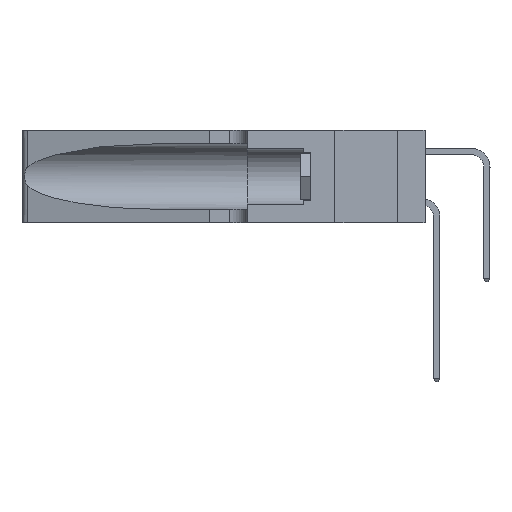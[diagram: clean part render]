
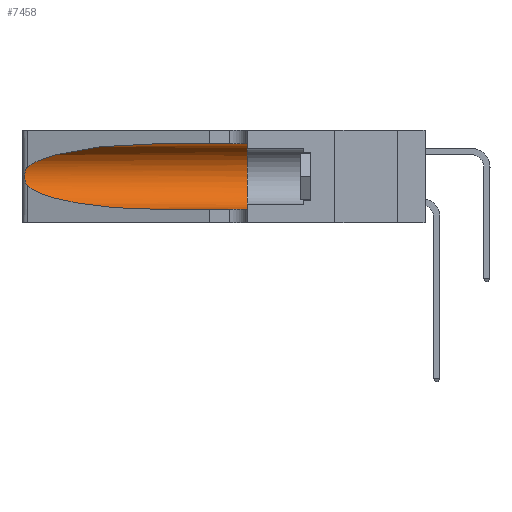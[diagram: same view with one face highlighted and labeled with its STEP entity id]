
A CAD part, left-side view. The second image highlights one B-rep face of the part: STEP entity #7458.
In plain terms, the highlighted cylindrical face has radius 3.308 mm (diameter 6.617 mm), a partial arc.
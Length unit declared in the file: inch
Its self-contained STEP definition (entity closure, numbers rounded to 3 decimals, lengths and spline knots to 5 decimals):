
#103 = CARTESIAN_POINT ( 'NONE',  ( 0.1305, 1.61858, 0.05475 ) ) ;
#185 = DIRECTION ( 'NONE',  ( 0., -1., 0. ) ) ;
#782 = B_SPLINE_CURVE_WITH_KNOTS ( 'NONE', 3,
 ( #19100, #15701, #3458, #15785, #5292, #17506, #7120, #19171, #8895, #20859, #10693, #22565, #12404, #1718 ),
 .UNSPECIFIED., .F., .F.,
 ( 4, 2, 2, 2, 2, 2, 4 ),
 ( 0., 0.00027, 0.00053, 0.00107, 0.0016, 0.00187, 0.00214 ),
 .UNSPECIFIED. ) ;
#835 = DIRECTION ( 'NONE',  ( 0., 0., -1. ) ) ;
#1412 = VERTEX_POINT ( 'NONE', #7590 ) ;
#1500 = CARTESIAN_POINT ( 'NONE',  ( 0.1305, 0.35, 0.31525 ) ) ;
#1718 = CARTESIAN_POINT ( 'NONE',  ( 0.25487, 1.22718, 0.14631 ) ) ;
#2585 = DIRECTION ( 'NONE',  ( 0., 1., 0. ) ) ;
#3244 =( BOUNDED_CURVE ( )  B_SPLINE_CURVE ( 3, ( #16791, #18538, #8221, #20223 ),
 .UNSPECIFIED., .F., .F. ) 
 B_SPLINE_CURVE_WITH_KNOTS ( ( 4, 4 ),
 ( 3.44316, 4.71239 ),
 .UNSPECIFIED. ) 
 CURVE ( )  GEOMETRIC_REPRESENTATION_ITEM ( )  RATIONAL_B_SPLINE_CURVE ( ( 1., 0.87, 0.87, 1. ) ) 
 REPRESENTATION_ITEM ( '' )  );
#3458 = CARTESIAN_POINT ( 'NONE',  ( 0.25639, 1.23184, 0.21858 ) ) ;
#3823 = EDGE_CURVE ( 'NONE', #5404, #13531, #11294, .T. ) ;
#4057 = EDGE_CURVE ( 'NONE', #19963, #5404, #20044, .T. ) ;
#4333 = EDGE_CURVE ( 'NONE', #20969, #13531, #15296, .T. ) ;
#4766 = CARTESIAN_POINT ( 'NONE',  ( 0.25487, 1.22718, 0.14631 ) ) ;
#4829 = CARTESIAN_POINT ( 'NONE',  ( 0.1305, 0.72297, 0.05475 ) ) ;
#4908 = ORIENTED_EDGE ( 'NONE', *, *, #4333, .T. ) ;
#4962 = DIRECTION ( 'NONE',  ( 0., -1., 0. ) ) ;
#5292 = CARTESIAN_POINT ( 'NONE',  ( 0.25854, 1.2359, 0.20912 ) ) ;
#5404 = VERTEX_POINT ( 'NONE', #1500 ) ;
#5486 = EDGE_CURVE ( 'NONE', #19963, #1412, #5718, .T. ) ;
#5718 =( BOUNDED_CURVE ( )  B_SPLINE_CURVE ( 3, ( #18509, #8193, #20181, #9987 ),
 .UNSPECIFIED., .F., .T. ) 
 B_SPLINE_CURVE_WITH_KNOTS ( ( 4, 4 ),
 ( 1.5708, 2.84003 ),
 .UNSPECIFIED. ) 
 CURVE ( )  GEOMETRIC_REPRESENTATION_ITEM ( )  RATIONAL_B_SPLINE_CURVE ( ( 1., 0.87, 0.87, 1. ) ) 
 REPRESENTATION_ITEM ( '' )  );
#6561 = VECTOR ( 'NONE', #185, 39.37008 ) ;
#6978 = ORIENTED_EDGE ( 'NONE', *, *, #3823, .F. ) ;
#7120 = CARTESIAN_POINT ( 'NONE',  ( 0.26075, 1.23896, 0.19203 ) ) ;
#7458 = ADVANCED_FACE ( 'NONE', ( #16131 ), #15579, .F. ) ;
#7590 = CARTESIAN_POINT ( 'NONE',  ( 0.25487, 1.22718, 0.22369 ) ) ;
#8193 = CARTESIAN_POINT ( 'NONE',  ( 0.18966, 0.96281, 0.31525 ) ) ;
#8221 = CARTESIAN_POINT ( 'NONE',  ( 0.18966, 0.96281, 0.05475 ) ) ;
#8895 = CARTESIAN_POINT ( 'NONE',  ( 0.26017, 1.23833, 0.17102 ) ) ;
#9668 = ORIENTED_EDGE ( 'NONE', *, *, #10316, .T. ) ;
#9823 = CARTESIAN_POINT ( 'NONE',  ( 0.1305, 0.72297, 0.31525 ) ) ;
#9987 = CARTESIAN_POINT ( 'NONE',  ( 0.25487, 1.22718, 0.22369 ) ) ;
#10316 = EDGE_CURVE ( 'NONE', #15887, #20969, #3244, .T. ) ;
#10693 = CARTESIAN_POINT ( 'NONE',  ( 0.25789, 1.23486, 0.15765 ) ) ;
#11294 = CIRCLE ( 'NONE', #16471, 0.13025 ) ;
#11566 = DIRECTION ( 'NONE',  ( 0., -1., 0. ) ) ;
#12404 = CARTESIAN_POINT ( 'NONE',  ( 0.25555, 1.22993, 0.14849 ) ) ;
#12434 = CARTESIAN_POINT ( 'NONE',  ( 0.1305, 0.35, 0.05475 ) ) ;
#13244 = CARTESIAN_POINT ( 'NONE',  ( 0.1305, 0.35, 0.185 ) ) ;
#13531 = VERTEX_POINT ( 'NONE', #12434 ) ;
#14082 = EDGE_CURVE ( 'NONE', #1412, #15887, #782, .T. ) ;
#14757 = EDGE_LOOP ( 'NONE', ( #18831, #22026, #9668, #4908, #6978, #21014 ) ) ;
#14878 = CARTESIAN_POINT ( 'NONE',  ( 0.1305, 1.61858, 0.185 ) ) ;
#14959 = DIRECTION ( 'NONE',  ( 0., 0., 1. ) ) ;
#15296 = LINE ( 'NONE', #103, #6561 ) ;
#15469 = CARTESIAN_POINT ( 'NONE',  ( 0.1305, 1.61858, 0.31525 ) ) ;
#15579 = CYLINDRICAL_SURFACE ( 'NONE', #17509, 0.13025 ) ;
#15701 = CARTESIAN_POINT ( 'NONE',  ( 0.25555, 1.22994, 0.2215 ) ) ;
#15785 = CARTESIAN_POINT ( 'NONE',  ( 0.25787, 1.23484, 0.2124 ) ) ;
#15887 = VERTEX_POINT ( 'NONE', #4766 ) ;
#16126 = VECTOR ( 'NONE', #4962, 39.37008 ) ;
#16131 = FACE_OUTER_BOUND ( 'NONE', #14757, .T. ) ;
#16471 = AXIS2_PLACEMENT_3D ( 'NONE', #13244, #2585, #14959 ) ;
#16791 = CARTESIAN_POINT ( 'NONE',  ( 0.25487, 1.22718, 0.14631 ) ) ;
#17506 = CARTESIAN_POINT ( 'NONE',  ( 0.26018, 1.23835, 0.19895 ) ) ;
#17509 = AXIS2_PLACEMENT_3D ( 'NONE', #14878, #11566, #835 ) ;
#18509 = CARTESIAN_POINT ( 'NONE',  ( 0.1305, 0.72297, 0.31525 ) ) ;
#18538 = CARTESIAN_POINT ( 'NONE',  ( 0.2373, 1.15595, 0.08982 ) ) ;
#18831 = ORIENTED_EDGE ( 'NONE', *, *, #5486, .T. ) ;
#19100 = CARTESIAN_POINT ( 'NONE',  ( 0.25487, 1.22718, 0.22369 ) ) ;
#19171 = CARTESIAN_POINT ( 'NONE',  ( 0.26075, 1.23896, 0.178 ) ) ;
#19963 = VERTEX_POINT ( 'NONE', #9823 ) ;
#20044 = LINE ( 'NONE', #15469, #16126 ) ;
#20181 = CARTESIAN_POINT ( 'NONE',  ( 0.2373, 1.15595, 0.28018 ) ) ;
#20223 = CARTESIAN_POINT ( 'NONE',  ( 0.1305, 0.72297, 0.05475 ) ) ;
#20859 = CARTESIAN_POINT ( 'NONE',  ( 0.25856, 1.23593, 0.16098 ) ) ;
#20969 = VERTEX_POINT ( 'NONE', #4829 ) ;
#21014 = ORIENTED_EDGE ( 'NONE', *, *, #4057, .F. ) ;
#22026 = ORIENTED_EDGE ( 'NONE', *, *, #14082, .T. ) ;
#22565 = CARTESIAN_POINT ( 'NONE',  ( 0.25639, 1.23186, 0.15144 ) ) ;
